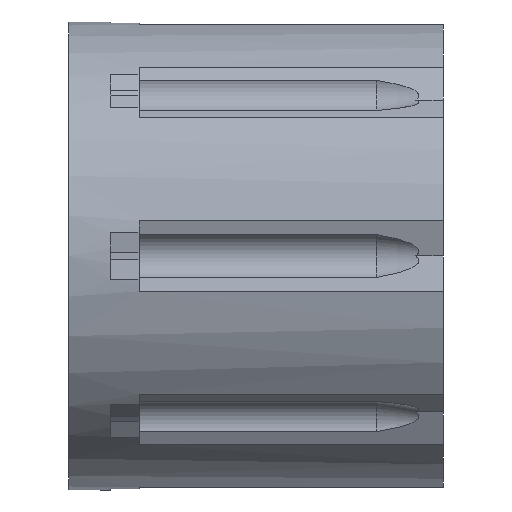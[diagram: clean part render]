
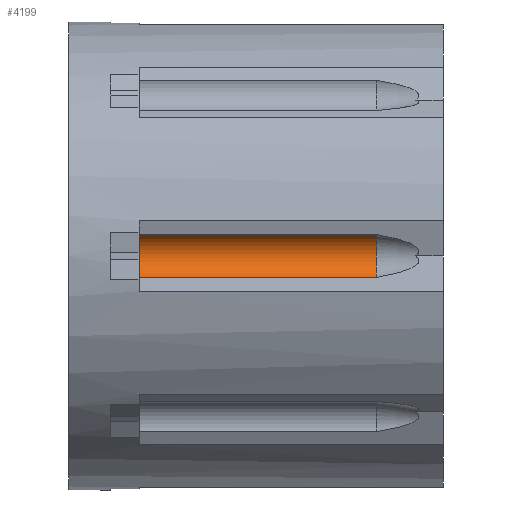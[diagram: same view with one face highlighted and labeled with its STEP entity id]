
A CAD part, front view. The second image highlights one B-rep face of the part: STEP entity #4199.
In plain terms, the highlighted cylindrical face has radius 5.1 mm (diameter 10.2 mm), a partial arc.
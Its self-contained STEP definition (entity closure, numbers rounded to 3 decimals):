
#131 = EDGE_CURVE ( 'NONE', #437, #2072, #783, .T. ) ;
#333 = VECTOR ( 'NONE', #2622, 1000. ) ;
#437 = VERTEX_POINT ( 'NONE', #3806 ) ;
#497 = DIRECTION ( 'NONE',  ( -1., 0., 0. ) ) ;
#783 = CIRCLE ( 'NONE', #3296, 5.1 ) ;
#1078 = VECTOR ( 'NONE', #1513, 1000. ) ;
#1187 = CARTESIAN_POINT ( 'NONE',  ( 15., -48.531, -4.592 ) ) ;
#1431 = CARTESIAN_POINT ( 'NONE',  ( 15., -48.531, -4.592 ) ) ;
#1495 = CARTESIAN_POINT ( 'NONE',  ( 65.715, -50.75, 0. ) ) ;
#1513 = DIRECTION ( 'NONE',  ( 1., 0., 0. ) ) ;
#1573 = ORIENTED_EDGE ( 'NONE', *, *, #4128, .T. ) ;
#1816 = EDGE_LOOP ( 'NONE', ( #2376, #1573, #4321, #1833 ) ) ;
#1833 = ORIENTED_EDGE ( 'NONE', *, *, #3766, .T. ) ;
#1841 = LINE ( 'NONE', #1187, #1078 ) ;
#1999 = CARTESIAN_POINT ( 'NONE',  ( 15., -50.75, 0. ) ) ;
#2072 = VERTEX_POINT ( 'NONE', #1431 ) ;
#2295 = DIRECTION ( 'NONE',  ( -1., 0., 0. ) ) ;
#2338 = DIRECTION ( 'NONE',  ( 0., 0., -1. ) ) ;
#2376 = ORIENTED_EDGE ( 'NONE', *, *, #131, .T. ) ;
#2551 = AXIS2_PLACEMENT_3D ( 'NONE', #4463, #2295, #2338 ) ;
#2599 = DIRECTION ( 'NONE',  ( 0., 0., -1. ) ) ;
#2607 = VERTEX_POINT ( 'NONE', #3628 ) ;
#2622 = DIRECTION ( 'NONE',  ( -1., 0., 0. ) ) ;
#2670 = EDGE_CURVE ( 'NONE', #2607, #4054, #2689, .T. ) ;
#2689 = CIRCLE ( 'NONE', #3813, 5.1 ) ;
#2964 = LINE ( 'NONE', #3697, #333 ) ;
#3095 = DIRECTION ( 'NONE',  ( -1., 0., 0. ) ) ;
#3296 = AXIS2_PLACEMENT_3D ( 'NONE', #1999, #3095, #4512 ) ;
#3314 = CARTESIAN_POINT ( 'NONE',  ( 65.715, -48.531, -4.592 ) ) ;
#3356 = CYLINDRICAL_SURFACE ( 'NONE', #2551, 5.1 ) ;
#3628 = CARTESIAN_POINT ( 'NONE',  ( 65.715, -48.531, 4.592 ) ) ;
#3697 = CARTESIAN_POINT ( 'NONE',  ( 15., -48.531, 4.592 ) ) ;
#3738 = FACE_OUTER_BOUND ( 'NONE', #1816, .T. ) ;
#3766 = EDGE_CURVE ( 'NONE', #2607, #437, #2964, .T. ) ;
#3806 = CARTESIAN_POINT ( 'NONE',  ( 15., -48.531, 4.592 ) ) ;
#3813 = AXIS2_PLACEMENT_3D ( 'NONE', #1495, #497, #2599 ) ;
#4054 = VERTEX_POINT ( 'NONE', #3314 ) ;
#4128 = EDGE_CURVE ( 'NONE', #2072, #4054, #1841, .T. ) ;
#4199 = ADVANCED_FACE ( 'NONE', ( #3738 ), #3356, .F. ) ;
#4321 = ORIENTED_EDGE ( 'NONE', *, *, #2670, .F. ) ;
#4463 = CARTESIAN_POINT ( 'NONE',  ( 15., -50.75, 0. ) ) ;
#4512 = DIRECTION ( 'NONE',  ( 0., 0., -1. ) ) ;
